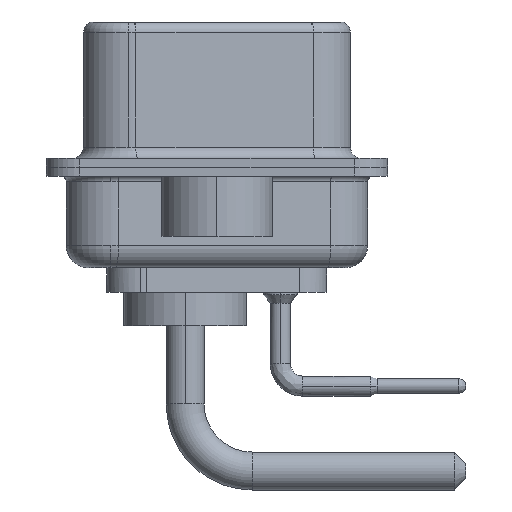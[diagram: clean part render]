
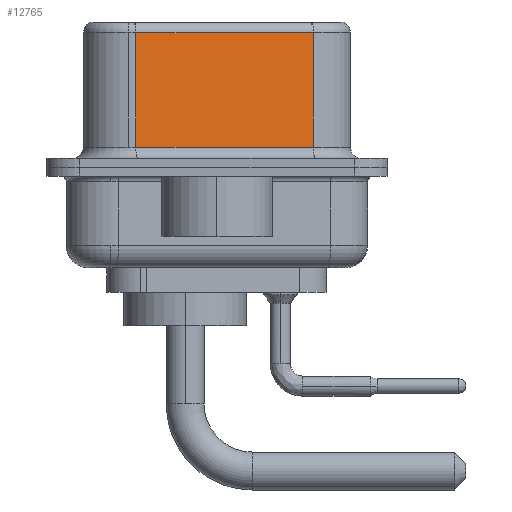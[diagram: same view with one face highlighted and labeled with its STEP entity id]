
A CAD part, left-side view. The second image highlights one B-rep face of the part: STEP entity #12765.
In plain terms, the highlighted planar face has unit normal (-0.985, -0.174, 0).
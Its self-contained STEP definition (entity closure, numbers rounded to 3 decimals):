
#1821 = DIRECTION ( 'NONE',  ( 0.174, -0.985, 0. ) ) ;
#2141 = CARTESIAN_POINT ( 'NONE',  ( 3.73, 3.628, 6.52 ) ) ;
#2326 = EDGE_LOOP ( 'NONE', ( #11905, #6283, #9498, #4048 ) ) ;
#4048 = ORIENTED_EDGE ( 'NONE', *, *, #13811, .T. ) ;
#4067 = CARTESIAN_POINT ( 'NONE',  ( 5.132, -4.322, 6.02 ) ) ;
#4484 = EDGE_CURVE ( 'NONE', #23091, #15750, #20527, .T. ) ;
#6283 = ORIENTED_EDGE ( 'NONE', *, *, #4484, .T. ) ;
#7690 = VERTEX_POINT ( 'NONE', #12858 ) ;
#8020 = CARTESIAN_POINT ( 'NONE',  ( 3.73, 3.628, 6.02 ) ) ;
#8760 = VECTOR ( 'NONE', #9140, 1000. ) ;
#9140 = DIRECTION ( 'NONE',  ( 0., 0., -1. ) ) ;
#9498 = ORIENTED_EDGE ( 'NONE', *, *, #18752, .T. ) ;
#9866 = DIRECTION ( 'NONE',  ( -0.174, 0.985, 0. ) ) ;
#10906 = CARTESIAN_POINT ( 'NONE',  ( 5.132, -4.322, 6.52 ) ) ;
#11317 = DIRECTION ( 'NONE',  ( -0.174, 0.985, 0. ) ) ;
#11518 = VECTOR ( 'NONE', #11317, 1000. ) ;
#11905 = ORIENTED_EDGE ( 'NONE', *, *, #19729, .F. ) ;
#12025 = DIRECTION ( 'NONE',  ( 0.985, 0.174, 0. ) ) ;
#12765 = ADVANCED_FACE ( 'NONE', ( #17357 ), #19402, .F. ) ;
#12858 = CARTESIAN_POINT ( 'NONE',  ( 3.73, 3.628, 0.9 ) ) ;
#13811 = EDGE_CURVE ( 'NONE', #7690, #14059, #15002, .T. ) ;
#14059 = VERTEX_POINT ( 'NONE', #22975 ) ;
#15002 = LINE ( 'NONE', #20330, #15525 ) ;
#15525 = VECTOR ( 'NONE', #1821, 1000. ) ;
#15750 = VERTEX_POINT ( 'NONE', #8020 ) ;
#16588 = LINE ( 'NONE', #10906, #17690 ) ;
#16763 = LINE ( 'NONE', #2141, #8760 ) ;
#17357 = FACE_OUTER_BOUND ( 'NONE', #2326, .T. ) ;
#17690 = VECTOR ( 'NONE', #20594, 1000. ) ;
#18633 = AXIS2_PLACEMENT_3D ( 'NONE', #22564, #12025, #9866 ) ;
#18752 = EDGE_CURVE ( 'NONE', #15750, #7690, #16763, .T. ) ;
#19402 = PLANE ( 'NONE',  #18633 ) ;
#19729 = EDGE_CURVE ( 'NONE', #23091, #14059, #16588, .T. ) ;
#20330 = CARTESIAN_POINT ( 'NONE',  ( 5.132, -4.322, 0.9 ) ) ;
#20527 = LINE ( 'NONE', #4067, #11518 ) ;
#20594 = DIRECTION ( 'NONE',  ( 0., 0., -1. ) ) ;
#22564 = CARTESIAN_POINT ( 'NONE',  ( 5.132, -4.322, 6.52 ) ) ;
#22975 = CARTESIAN_POINT ( 'NONE',  ( 5.132, -4.322, 0.9 ) ) ;
#23091 = VERTEX_POINT ( 'NONE', #23820 ) ;
#23820 = CARTESIAN_POINT ( 'NONE',  ( 5.132, -4.322, 6.02 ) ) ;
